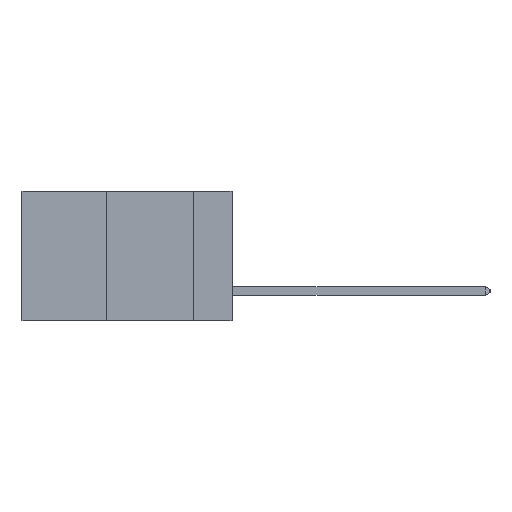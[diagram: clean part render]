
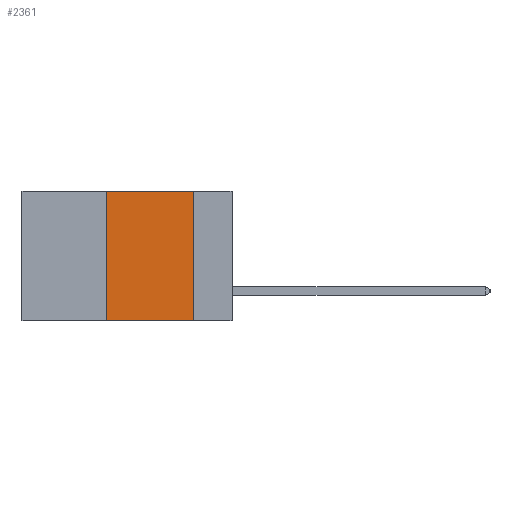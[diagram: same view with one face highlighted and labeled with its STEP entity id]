
A CAD part, left-side view. The second image highlights one B-rep face of the part: STEP entity #2361.
In plain terms, the highlighted planar face has unit normal (-1, 0, 0).
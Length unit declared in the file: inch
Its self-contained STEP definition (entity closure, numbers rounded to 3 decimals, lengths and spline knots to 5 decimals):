
#581 = ORIENTED_EDGE ( 'NONE', *, *, #9114, .F. ) ;
#639 = CARTESIAN_POINT ( 'NONE',  ( 0., 0.11, 0. ) ) ;
#1688 = VECTOR ( 'NONE', #12686, 39.37008 ) ;
#2361 = ADVANCED_FACE ( 'NONE', ( #6325 ), #5885, .F. ) ;
#2875 = VERTEX_POINT ( 'NONE', #23158 ) ;
#3482 = CARTESIAN_POINT ( 'NONE',  ( 0., 0.11, -0.37 ) ) ;
#4155 = VERTEX_POINT ( 'NONE', #16594 ) ;
#4221 = VERTEX_POINT ( 'NONE', #24637 ) ;
#4885 = AXIS2_PLACEMENT_3D ( 'NONE', #21643, #9816, #23622 ) ;
#5047 = VERTEX_POINT ( 'NONE', #3482 ) ;
#5885 = PLANE ( 'NONE',  #4885 ) ;
#6325 = FACE_OUTER_BOUND ( 'NONE', #21707, .T. ) ;
#8358 = DIRECTION ( 'NONE',  ( 0., -1., 0. ) ) ;
#9068 = VECTOR ( 'NONE', #20883, 39.37008 ) ;
#9114 = EDGE_CURVE ( 'NONE', #4155, #2875, #19588, .T. ) ;
#9816 = DIRECTION ( 'NONE',  ( 1., 0., 0. ) ) ;
#9827 = ORIENTED_EDGE ( 'NONE', *, *, #22474, .F. ) ;
#9950 = VECTOR ( 'NONE', #8358, 39.37008 ) ;
#10935 = EDGE_CURVE ( 'NONE', #4221, #5047, #22227, .T. ) ;
#11087 = ORIENTED_EDGE ( 'NONE', *, *, #15278, .T. ) ;
#12686 = DIRECTION ( 'NONE',  ( 0., -1., 0. ) ) ;
#14628 = LINE ( 'NONE', #20175, #9950 ) ;
#15278 = EDGE_CURVE ( 'NONE', #4155, #5047, #14628, .T. ) ;
#16594 = CARTESIAN_POINT ( 'NONE',  ( 0., 0.36, -0.37 ) ) ;
#17043 = VECTOR ( 'NONE', #18425, 39.37008 ) ;
#18425 = DIRECTION ( 'NONE',  ( 0., 0., -1. ) ) ;
#18931 = CARTESIAN_POINT ( 'NONE',  ( 0., 0.36, 0. ) ) ;
#19588 = LINE ( 'NONE', #18931, #9068 ) ;
#20175 = CARTESIAN_POINT ( 'NONE',  ( 0., 0.6, -0.37 ) ) ;
#20883 = DIRECTION ( 'NONE',  ( 0., 0., 1. ) ) ;
#21643 = CARTESIAN_POINT ( 'NONE',  ( 0., 0.6, 0. ) ) ;
#21707 = EDGE_LOOP ( 'NONE', ( #24939, #9827, #581, #11087 ) ) ;
#22227 = LINE ( 'NONE', #639, #17043 ) ;
#22463 = CARTESIAN_POINT ( 'NONE',  ( 0., 0.6, 0. ) ) ;
#22474 = EDGE_CURVE ( 'NONE', #2875, #4221, #22652, .T. ) ;
#22652 = LINE ( 'NONE', #22463, #1688 ) ;
#23158 = CARTESIAN_POINT ( 'NONE',  ( 0., 0.36, 0. ) ) ;
#23622 = DIRECTION ( 'NONE',  ( 0., 0., -1. ) ) ;
#24637 = CARTESIAN_POINT ( 'NONE',  ( 0., 0.11, 0. ) ) ;
#24939 = ORIENTED_EDGE ( 'NONE', *, *, #10935, .F. ) ;
